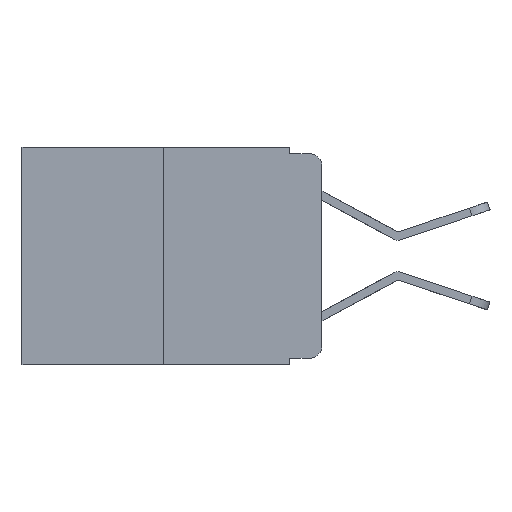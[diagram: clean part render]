
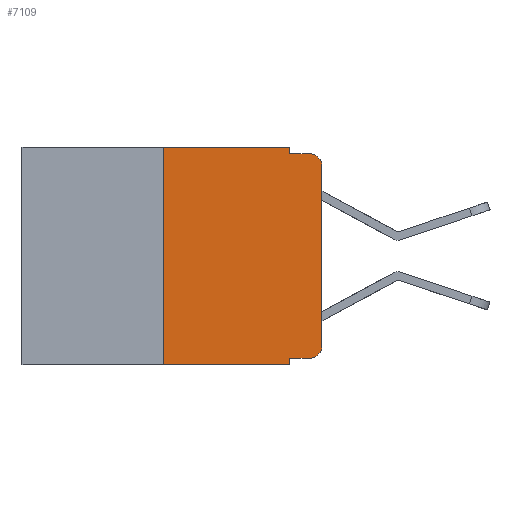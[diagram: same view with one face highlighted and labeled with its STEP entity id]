
A CAD part, left-side view. The second image highlights one B-rep face of the part: STEP entity #7109.
In plain terms, the highlighted planar face has unit normal (-1, 0, 0).
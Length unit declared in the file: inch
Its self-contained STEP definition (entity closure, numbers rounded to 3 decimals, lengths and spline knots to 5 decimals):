
#148 = CARTESIAN_POINT ( 'NONE',  ( 0., 0., -0.03 ) ) ;
#516 = PLANE ( 'NONE',  #17680 ) ;
#969 = LINE ( 'NONE', #3544, #15895 ) ;
#1197 = ORIENTED_EDGE ( 'NONE', *, *, #16174, .T. ) ;
#1198 = CARTESIAN_POINT ( 'NONE',  ( 0., 0.25, 0. ) ) ;
#1206 = CARTESIAN_POINT ( 'NONE',  ( 0., 0.473, 0. ) ) ;
#1490 = EDGE_LOOP ( 'NONE', ( #16400, #7439, #23138, #3417, #4041, #5271, #1197, #22272, #2492, #3117 ) ) ;
#1628 = VERTEX_POINT ( 'NONE', #4408 ) ;
#2156 = VERTEX_POINT ( 'NONE', #10450 ) ;
#2492 = ORIENTED_EDGE ( 'NONE', *, *, #14276, .T. ) ;
#2631 = CARTESIAN_POINT ( 'NONE',  ( 0., 0.051, 0. ) ) ;
#2838 = CARTESIAN_POINT ( 'NONE',  ( 0., 0.051, -0.333 ) ) ;
#3117 = ORIENTED_EDGE ( 'NONE', *, *, #10475, .T. ) ;
#3417 = ORIENTED_EDGE ( 'NONE', *, *, #18560, .F. ) ;
#3544 = CARTESIAN_POINT ( 'NONE',  ( 0., 0.051, -0.333 ) ) ;
#3797 = VERTEX_POINT ( 'NONE', #148 ) ;
#3835 = LINE ( 'NONE', #1206, #17969 ) ;
#4041 = ORIENTED_EDGE ( 'NONE', *, *, #7857, .F. ) ;
#4408 = CARTESIAN_POINT ( 'NONE',  ( 0., 0., -0.313 ) ) ;
#5000 = DIRECTION ( 'NONE',  ( 0., 0., -1. ) ) ;
#5016 = CARTESIAN_POINT ( 'NONE',  ( 0., 0.051, -0.01 ) ) ;
#5207 = LINE ( 'NONE', #5016, #24809 ) ;
#5234 = DIRECTION ( 'NONE',  ( 0., 0., 1. ) ) ;
#5237 = EDGE_CURVE ( 'NONE', #7720, #9634, #17272, .T. ) ;
#5271 = ORIENTED_EDGE ( 'NONE', *, *, #7887, .F. ) ;
#5676 = CARTESIAN_POINT ( 'NONE',  ( 0., 0.02, -0.313 ) ) ;
#5889 = VERTEX_POINT ( 'NONE', #1198 ) ;
#6475 = CARTESIAN_POINT ( 'NONE',  ( 0., 0.051, -0.343 ) ) ;
#6534 = CARTESIAN_POINT ( 'NONE',  ( 0., 0.473, 0. ) ) ;
#7109 = ADVANCED_FACE ( 'NONE', ( #18561 ), #516, .F. ) ;
#7439 = ORIENTED_EDGE ( 'NONE', *, *, #17315, .T. ) ;
#7687 = DIRECTION ( 'NONE',  ( 0., 0., -1. ) ) ;
#7720 = VERTEX_POINT ( 'NONE', #2838 ) ;
#7778 = CIRCLE ( 'NONE', #16131, 0.02 ) ;
#7857 = EDGE_CURVE ( 'NONE', #5889, #10050, #3835, .T. ) ;
#7887 = EDGE_CURVE ( 'NONE', #2156, #5889, #18566, .T. ) ;
#8522 = DIRECTION ( 'NONE',  ( 0., 0., -1. ) ) ;
#9157 = CARTESIAN_POINT ( 'NONE',  ( 0., 0., 0. ) ) ;
#9634 = VERTEX_POINT ( 'NONE', #6475 ) ;
#9968 = CARTESIAN_POINT ( 'NONE',  ( 0., 0.02, -0.03 ) ) ;
#10050 = VERTEX_POINT ( 'NONE', #17371 ) ;
#10275 = CARTESIAN_POINT ( 'NONE',  ( 0., 0.473, -0.343 ) ) ;
#10450 = CARTESIAN_POINT ( 'NONE',  ( 0., 0.25, -0.343 ) ) ;
#10475 = EDGE_CURVE ( 'NONE', #15108, #1628, #11341, .T. ) ;
#11099 = DIRECTION ( 'NONE',  ( 0., 0., 1. ) ) ;
#11118 = CARTESIAN_POINT ( 'NONE',  ( 0., 0.25, 0. ) ) ;
#11341 = CIRCLE ( 'NONE', #16156, 0.02 ) ;
#11884 = DIRECTION ( 'NONE',  ( 0., 0., -1. ) ) ;
#12178 = DIRECTION ( 'NONE',  ( 0., -1., 0. ) ) ;
#12211 = VECTOR ( 'NONE', #5000, 39.37008 ) ;
#12694 = CARTESIAN_POINT ( 'NONE',  ( 0., 0.051, 0. ) ) ;
#12767 = VECTOR ( 'NONE', #18043, 39.37008 ) ;
#12912 = VECTOR ( 'NONE', #5234, 39.37008 ) ;
#13367 = LINE ( 'NONE', #2631, #12767 ) ;
#13465 = EDGE_CURVE ( 'NONE', #1628, #3797, #24143, .T. ) ;
#14276 = EDGE_CURVE ( 'NONE', #7720, #15108, #969, .T. ) ;
#15108 = VERTEX_POINT ( 'NONE', #23254 ) ;
#15895 = VECTOR ( 'NONE', #17040, 39.37008 ) ;
#16131 = AXIS2_PLACEMENT_3D ( 'NONE', #9968, #23160, #11884 ) ;
#16156 = AXIS2_PLACEMENT_3D ( 'NONE', #5676, #19099, #7687 ) ;
#16174 = EDGE_CURVE ( 'NONE', #2156, #9634, #18860, .T. ) ;
#16400 = ORIENTED_EDGE ( 'NONE', *, *, #13465, .T. ) ;
#17040 = DIRECTION ( 'NONE',  ( 0., -1., 0. ) ) ;
#17082 = VECTOR ( 'NONE', #12178, 39.37008 ) ;
#17272 = LINE ( 'NONE', #12694, #12211 ) ;
#17315 = EDGE_CURVE ( 'NONE', #3797, #17555, #7778, .T. ) ;
#17371 = CARTESIAN_POINT ( 'NONE',  ( 0., 0.051, 0. ) ) ;
#17555 = VERTEX_POINT ( 'NONE', #18588 ) ;
#17680 = AXIS2_PLACEMENT_3D ( 'NONE', #6534, #19921, #8522 ) ;
#17969 = VECTOR ( 'NONE', #22241, 39.37008 ) ;
#18043 = DIRECTION ( 'NONE',  ( 0., 0., -1. ) ) ;
#18438 = DIRECTION ( 'NONE',  ( 0., -1., 0. ) ) ;
#18560 = EDGE_CURVE ( 'NONE', #10050, #24807, #13367, .T. ) ;
#18561 = FACE_OUTER_BOUND ( 'NONE', #1490, .T. ) ;
#18566 = LINE ( 'NONE', #11118, #12912 ) ;
#18588 = CARTESIAN_POINT ( 'NONE',  ( 0., 0.02, -0.01 ) ) ;
#18860 = LINE ( 'NONE', #10275, #17082 ) ;
#19099 = DIRECTION ( 'NONE',  ( -1., 0., 0. ) ) ;
#19921 = DIRECTION ( 'NONE',  ( 1., 0., 0. ) ) ;
#22120 = CARTESIAN_POINT ( 'NONE',  ( 0., 0.051, -0.01 ) ) ;
#22241 = DIRECTION ( 'NONE',  ( 0., -1., 0. ) ) ;
#22272 = ORIENTED_EDGE ( 'NONE', *, *, #5237, .F. ) ;
#23138 = ORIENTED_EDGE ( 'NONE', *, *, #24800, .F. ) ;
#23160 = DIRECTION ( 'NONE',  ( -1., 0., 0. ) ) ;
#23254 = CARTESIAN_POINT ( 'NONE',  ( 0., 0.02, -0.333 ) ) ;
#24143 = LINE ( 'NONE', #9157, #24713 ) ;
#24713 = VECTOR ( 'NONE', #11099, 39.37008 ) ;
#24800 = EDGE_CURVE ( 'NONE', #24807, #17555, #5207, .T. ) ;
#24807 = VERTEX_POINT ( 'NONE', #22120 ) ;
#24809 = VECTOR ( 'NONE', #18438, 39.37008 ) ;
